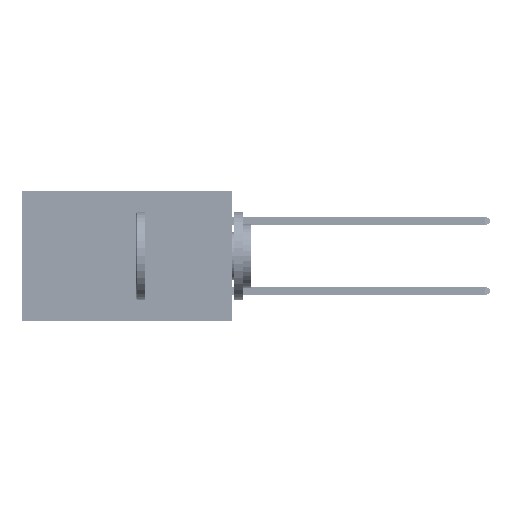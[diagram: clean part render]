
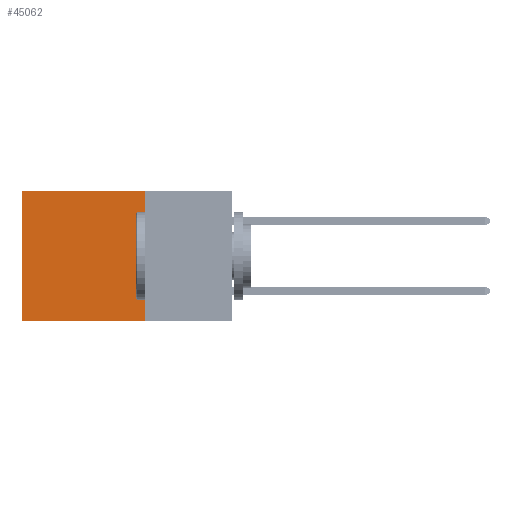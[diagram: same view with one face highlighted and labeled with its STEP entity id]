
A CAD part, left-side view. The second image highlights one B-rep face of the part: STEP entity #45062.
In plain terms, the highlighted planar face has unit normal (-1, 0, 0).
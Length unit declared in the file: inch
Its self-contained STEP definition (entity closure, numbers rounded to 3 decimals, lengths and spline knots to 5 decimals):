
#214 = LINE ( 'NONE', #21688, #18199 ) ;
#1245 = VERTEX_POINT ( 'NONE', #26883 ) ;
#6330 = CARTESIAN_POINT ( 'NONE',  ( 0.2875, 0.25, 0. ) ) ;
#6467 = CARTESIAN_POINT ( 'NONE',  ( 0.2875, 0.25, -0.37 ) ) ;
#7820 = LINE ( 'NONE', #23382, #47359 ) ;
#10588 = CARTESIAN_POINT ( 'NONE',  ( 0.2875, 0.25, 0. ) ) ;
#10819 = ORIENTED_EDGE ( 'NONE', *, *, #32839, .T. ) ;
#11897 = CARTESIAN_POINT ( 'NONE',  ( 0.2875, 0.6, 0. ) ) ;
#12697 = EDGE_CURVE ( 'NONE', #36703, #28990, #34198, .T. ) ;
#14162 = DIRECTION ( 'NONE',  ( 0., 0., -1. ) ) ;
#15652 = DIRECTION ( 'NONE',  ( 0., 1., 0. ) ) ;
#15664 = ORIENTED_EDGE ( 'NONE', *, *, #12697, .F. ) ;
#16646 = EDGE_CURVE ( 'NONE', #36703, #1245, #7820, .T. ) ;
#18199 = VECTOR ( 'NONE', #41187, 39.37008 ) ;
#18295 = PLANE ( 'NONE',  #36495 ) ;
#20884 = FACE_OUTER_BOUND ( 'NONE', #40467, .T. ) ;
#21688 = CARTESIAN_POINT ( 'NONE',  ( 0.2875, 0.25, -0.37 ) ) ;
#21849 = VERTEX_POINT ( 'NONE', #33044 ) ;
#23382 = CARTESIAN_POINT ( 'NONE',  ( 0.2875, 0.25, 0. ) ) ;
#26883 = CARTESIAN_POINT ( 'NONE',  ( 0.2875, 0.6, 0. ) ) ;
#28990 = VERTEX_POINT ( 'NONE', #6467 ) ;
#30980 = CARTESIAN_POINT ( 'NONE',  ( 0.2875, 0.25, 0. ) ) ;
#31731 = DIRECTION ( 'NONE',  ( 0., 0., -1. ) ) ;
#32839 = EDGE_CURVE ( 'NONE', #1245, #21849, #42854, .T. ) ;
#33044 = CARTESIAN_POINT ( 'NONE',  ( 0.2875, 0.6, -0.37 ) ) ;
#33089 = EDGE_CURVE ( 'NONE', #28990, #21849, #214, .T. ) ;
#34198 = LINE ( 'NONE', #30980, #38422 ) ;
#36495 = AXIS2_PLACEMENT_3D ( 'NONE', #6330, #42060, #14162 ) ;
#36703 = VERTEX_POINT ( 'NONE', #10588 ) ;
#37303 = VECTOR ( 'NONE', #31731, 39.37008 ) ;
#38422 = VECTOR ( 'NONE', #47051, 39.37008 ) ;
#40467 = EDGE_LOOP ( 'NONE', ( #10819, #50190, #15664, #45611 ) ) ;
#41187 = DIRECTION ( 'NONE',  ( 0., 1., 0. ) ) ;
#42060 = DIRECTION ( 'NONE',  ( 1., 0., 0. ) ) ;
#42854 = LINE ( 'NONE', #11897, #37303 ) ;
#45062 = ADVANCED_FACE ( 'NONE', ( #20884 ), #18295, .F. ) ;
#45611 = ORIENTED_EDGE ( 'NONE', *, *, #16646, .T. ) ;
#47051 = DIRECTION ( 'NONE',  ( 0., 0., -1. ) ) ;
#47359 = VECTOR ( 'NONE', #15652, 39.37008 ) ;
#50190 = ORIENTED_EDGE ( 'NONE', *, *, #33089, .F. ) ;
